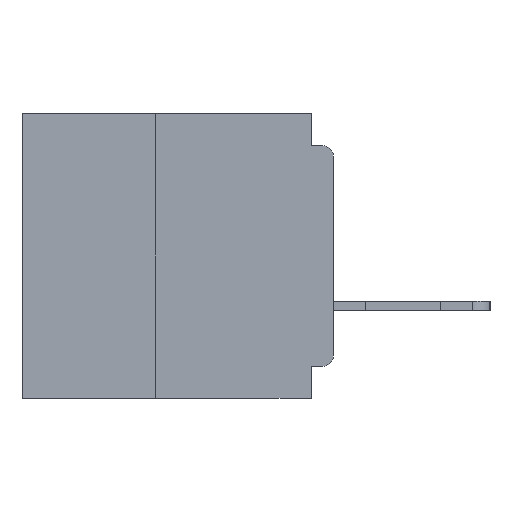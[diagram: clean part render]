
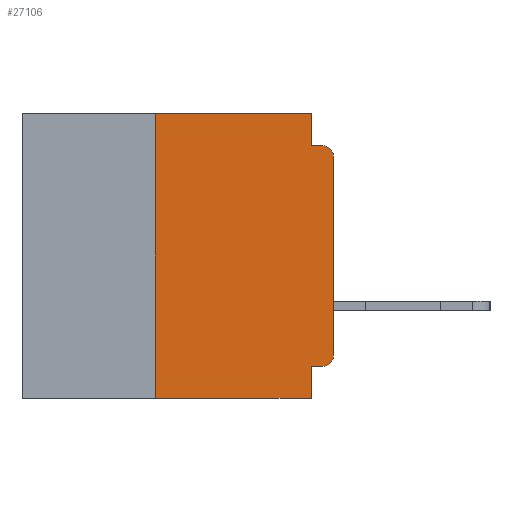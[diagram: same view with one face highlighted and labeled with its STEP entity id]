
A CAD part, left-side view. The second image highlights one B-rep face of the part: STEP entity #27106.
In plain terms, the highlighted planar face has unit normal (-1, 0, 0).
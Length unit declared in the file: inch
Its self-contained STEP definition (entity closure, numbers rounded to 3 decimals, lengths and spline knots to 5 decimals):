
#1260 = CARTESIAN_POINT ( 'NONE',  ( 0., 0.031, -0.045 ) ) ;
#1463 = LINE ( 'NONE', #48511, #41396 ) ;
#1656 = EDGE_CURVE ( 'NONE', #19831, #46139, #7005, .T. ) ;
#2000 = VERTEX_POINT ( 'NONE', #1260 ) ;
#2233 = EDGE_CURVE ( 'NONE', #26820, #2000, #31013, .T. ) ;
#2450 = AXIS2_PLACEMENT_3D ( 'NONE', #27615, #5124, #31354 ) ;
#3054 = LINE ( 'NONE', #20196, #30630 ) ;
#3340 = CARTESIAN_POINT ( 'NONE',  ( 0., 0.031, 0. ) ) ;
#3354 = CARTESIAN_POINT ( 'NONE',  ( 0., 0., 0. ) ) ;
#4657 = LINE ( 'NONE', #3354, #33447 ) ;
#4687 = CARTESIAN_POINT ( 'NONE',  ( 0., 0.25, 0. ) ) ;
#5124 = DIRECTION ( 'NONE',  ( 1., 0., 0. ) ) ;
#5138 = DIRECTION ( 'NONE',  ( -1., 0., 0. ) ) ;
#6395 = LINE ( 'NONE', #34371, #45158 ) ;
#7005 = CIRCLE ( 'NONE', #10778, 0.015 ) ;
#7186 = EDGE_CURVE ( 'NONE', #39230, #28532, #37698, .T. ) ;
#9140 = FACE_OUTER_BOUND ( 'NONE', #42090, .T. ) ;
#9648 = CIRCLE ( 'NONE', #31033, 0.015 ) ;
#10778 = AXIS2_PLACEMENT_3D ( 'NONE', #21845, #21576, #21100 ) ;
#11868 = DIRECTION ( 'NONE',  ( 0., -1., 0. ) ) ;
#12357 = ORIENTED_EDGE ( 'NONE', *, *, #1656, .T. ) ;
#12365 = EDGE_CURVE ( 'NONE', #24957, #33817, #41871, .T. ) ;
#12681 = ORIENTED_EDGE ( 'NONE', *, *, #17558, .T. ) ;
#12876 = CARTESIAN_POINT ( 'NONE',  ( 0., 0., -0.06 ) ) ;
#14166 = CARTESIAN_POINT ( 'NONE',  ( 0., 0.25, -0.4 ) ) ;
#14322 = ORIENTED_EDGE ( 'NONE', *, *, #25186, .F. ) ;
#14750 = CARTESIAN_POINT ( 'NONE',  ( 0., 0.25, -0.4 ) ) ;
#15228 = ORIENTED_EDGE ( 'NONE', *, *, #12365, .F. ) ;
#15270 = DIRECTION ( 'NONE',  ( 0., 0., -1. ) ) ;
#17558 = EDGE_CURVE ( 'NONE', #42042, #33630, #9648, .T. ) ;
#18575 = DIRECTION ( 'NONE',  ( 0., 0., 1. ) ) ;
#19831 = VERTEX_POINT ( 'NONE', #20188 ) ;
#20188 = CARTESIAN_POINT ( 'NONE',  ( 0., 0.015, -0.355 ) ) ;
#20196 = CARTESIAN_POINT ( 'NONE',  ( 0., 0.437, -0.4 ) ) ;
#21100 = DIRECTION ( 'NONE',  ( 0., 0., -1. ) ) ;
#21576 = DIRECTION ( 'NONE',  ( -1., 0., 0. ) ) ;
#21845 = CARTESIAN_POINT ( 'NONE',  ( 0., 0.015, -0.34 ) ) ;
#21907 = VECTOR ( 'NONE', #18575, 39.37008 ) ;
#23197 = CARTESIAN_POINT ( 'NONE',  ( 0., 0.031, -0.4 ) ) ;
#23955 = EDGE_CURVE ( 'NONE', #33817, #26820, #25335, .T. ) ;
#24170 = VECTOR ( 'NONE', #44622, 39.37008 ) ;
#24957 = VERTEX_POINT ( 'NONE', #14166 ) ;
#25046 = EDGE_CURVE ( 'NONE', #46139, #42042, #4657, .T. ) ;
#25186 = EDGE_CURVE ( 'NONE', #2000, #33630, #6395, .T. ) ;
#25335 = LINE ( 'NONE', #40855, #24170 ) ;
#26104 = DIRECTION ( 'NONE',  ( 0., 1., 0. ) ) ;
#26545 = VECTOR ( 'NONE', #15270, 39.37008 ) ;
#26820 = VERTEX_POINT ( 'NONE', #3340 ) ;
#27106 = ADVANCED_FACE ( 'NONE', ( #9140 ), #27442, .F. ) ;
#27442 = PLANE ( 'NONE',  #2450 ) ;
#27615 = CARTESIAN_POINT ( 'NONE',  ( 0., 0.437, 0. ) ) ;
#27629 = CARTESIAN_POINT ( 'NONE',  ( 0., 0.015, -0.06 ) ) ;
#28465 = ORIENTED_EDGE ( 'NONE', *, *, #25046, .T. ) ;
#28532 = VERTEX_POINT ( 'NONE', #23197 ) ;
#28948 = DIRECTION ( 'NONE',  ( 0., 0., -1. ) ) ;
#29269 = ORIENTED_EDGE ( 'NONE', *, *, #7186, .F. ) ;
#29958 = CARTESIAN_POINT ( 'NONE',  ( 0., 0.015, -0.045 ) ) ;
#30201 = CARTESIAN_POINT ( 'NONE',  ( 0., 0.031, -0.4 ) ) ;
#30630 = VECTOR ( 'NONE', #42666, 39.37008 ) ;
#31013 = LINE ( 'NONE', #40112, #48558 ) ;
#31033 = AXIS2_PLACEMENT_3D ( 'NONE', #27629, #5138, #31366 ) ;
#31354 = DIRECTION ( 'NONE',  ( 0., 0., -1. ) ) ;
#31366 = DIRECTION ( 'NONE',  ( 0., 0., -1. ) ) ;
#31756 = EDGE_CURVE ( 'NONE', #19831, #39230, #1463, .T. ) ;
#33240 = EDGE_CURVE ( 'NONE', #24957, #28532, #3054, .T. ) ;
#33447 = VECTOR ( 'NONE', #48243, 39.37008 ) ;
#33630 = VERTEX_POINT ( 'NONE', #29958 ) ;
#33720 = ORIENTED_EDGE ( 'NONE', *, *, #23955, .F. ) ;
#33817 = VERTEX_POINT ( 'NONE', #4687 ) ;
#34371 = CARTESIAN_POINT ( 'NONE',  ( 0., 0., -0.045 ) ) ;
#36648 = ORIENTED_EDGE ( 'NONE', *, *, #33240, .T. ) ;
#36800 = ORIENTED_EDGE ( 'NONE', *, *, #2233, .F. ) ;
#37698 = LINE ( 'NONE', #30201, #26545 ) ;
#39230 = VERTEX_POINT ( 'NONE', #42250 ) ;
#40108 = CARTESIAN_POINT ( 'NONE',  ( 0., 0., -0.34 ) ) ;
#40112 = CARTESIAN_POINT ( 'NONE',  ( 0., 0.031, 0. ) ) ;
#40855 = CARTESIAN_POINT ( 'NONE',  ( 0., 0.437, 0. ) ) ;
#41396 = VECTOR ( 'NONE', #26104, 39.37008 ) ;
#41871 = LINE ( 'NONE', #14750, #21907 ) ;
#42042 = VERTEX_POINT ( 'NONE', #12876 ) ;
#42090 = EDGE_LOOP ( 'NONE', ( #28465, #12681, #14322, #36800, #33720, #15228, #36648, #29269, #45323, #12357 ) ) ;
#42250 = CARTESIAN_POINT ( 'NONE',  ( 0., 0.031, -0.355 ) ) ;
#42666 = DIRECTION ( 'NONE',  ( 0., -1., 0. ) ) ;
#44622 = DIRECTION ( 'NONE',  ( 0., -1., 0. ) ) ;
#45158 = VECTOR ( 'NONE', #11868, 39.37008 ) ;
#45323 = ORIENTED_EDGE ( 'NONE', *, *, #31756, .F. ) ;
#46139 = VERTEX_POINT ( 'NONE', #40108 ) ;
#48243 = DIRECTION ( 'NONE',  ( 0., 0., 1. ) ) ;
#48511 = CARTESIAN_POINT ( 'NONE',  ( 0., 0., -0.355 ) ) ;
#48558 = VECTOR ( 'NONE', #28948, 39.37008 ) ;
